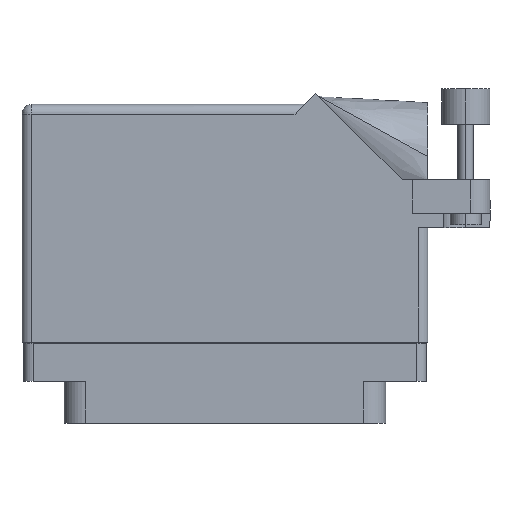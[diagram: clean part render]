
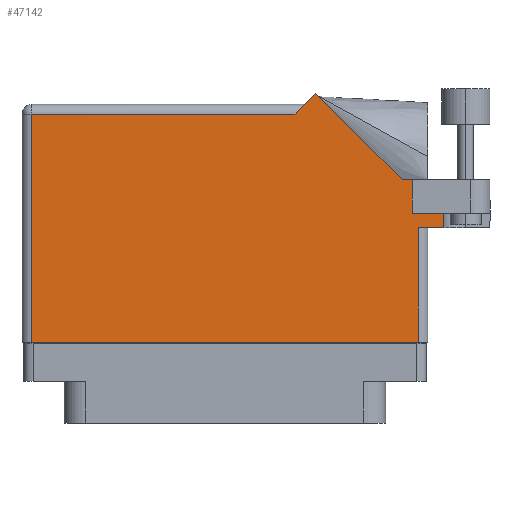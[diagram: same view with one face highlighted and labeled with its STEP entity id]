
A CAD part, front view. The second image highlights one B-rep face of the part: STEP entity #47142.
In plain terms, the highlighted face is planar.
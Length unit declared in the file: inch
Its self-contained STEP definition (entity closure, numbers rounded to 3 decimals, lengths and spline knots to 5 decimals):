
#153 = CARTESIAN_POINT ( 'NONE',  ( 1.206, 0.731, 0.455 ) ) ;
#438 = VERTEX_POINT ( 'NONE', #41555 ) ;
#1408 = LINE ( 'NONE', #45483, #38787 ) ;
#1766 = ORIENTED_EDGE ( 'NONE', *, *, #2080, .F. ) ;
#2080 = EDGE_CURVE ( 'NONE', #27989, #13766, #20685, .T. ) ;
#2596 = LINE ( 'NONE', #15896, #49463 ) ;
#3850 = VECTOR ( 'NONE', #30652, 39.37008 ) ;
#4051 = CARTESIAN_POINT ( 'NONE',  ( -1.244, 1.368, 0.455 ) ) ;
#4260 = EDGE_CURVE ( 'NONE', #438, #21775, #40558, .T. ) ;
#4798 = DIRECTION ( 'NONE',  ( 0., 0., -1. ) ) ;
#4998 = DIRECTION ( 'NONE',  ( -1., 0., 0. ) ) ;
#6506 = VECTOR ( 'NONE', #30229, 39.37008 ) ;
#7377 = LINE ( 'NONE', #37562, #49171 ) ;
#8509 = VERTEX_POINT ( 'NONE', #31426 ) ;
#9942 = EDGE_CURVE ( 'NONE', #13766, #21775, #1408, .T. ) ;
#10241 = VERTEX_POINT ( 'NONE', #4051 ) ;
#10254 = LINE ( 'NONE', #26733, #33143 ) ;
#10369 = CARTESIAN_POINT ( 'NONE',  ( -1.306, 1.368, 0.455 ) ) ;
#10616 = CARTESIAN_POINT ( 'NONE',  ( 1.14042, 0.944, 0.455 ) ) ;
#10882 = EDGE_CURVE ( 'NONE', #38971, #8509, #43104, .T. ) ;
#10927 = CARTESIAN_POINT ( 'NONE',  ( 0.451, 1.368, 0.455 ) ) ;
#11291 = EDGE_CURVE ( 'NONE', #8509, #37565, #29175, .T. ) ;
#12112 = ORIENTED_EDGE ( 'NONE', *, *, #28509, .T. ) ;
#13766 = VERTEX_POINT ( 'NONE', #40806 ) ;
#15241 = EDGE_CURVE ( 'NONE', #31106, #37190, #10254, .T. ) ;
#15896 = CARTESIAN_POINT ( 'NONE',  ( 1.244, 0.637, 0.455 ) ) ;
#17010 = DIRECTION ( 'NONE',  ( -1., 0., 0. ) ) ;
#17446 = CARTESIAN_POINT ( 'NONE',  ( 1.4075, 0.637, 0.455 ) ) ;
#17551 = DIRECTION ( 'NONE',  ( 1., 0., 0. ) ) ;
#18924 = VERTEX_POINT ( 'NONE', #46451 ) ;
#19337 = EDGE_CURVE ( 'NONE', #18924, #38971, #7377, .T. ) ;
#20122 = ORIENTED_EDGE ( 'NONE', *, *, #4260, .T. ) ;
#20175 = CARTESIAN_POINT ( 'NONE',  ( 1.244, -0.1, 0.455 ) ) ;
#20685 = LINE ( 'NONE', #153, #29537 ) ;
#21068 = ORIENTED_EDGE ( 'NONE', *, *, #10882, .T. ) ;
#21775 = VERTEX_POINT ( 'NONE', #17446 ) ;
#22113 = CARTESIAN_POINT ( 'NONE',  ( 1.306, 0.637, 0.455 ) ) ;
#22409 = LINE ( 'NONE', #50147, #35077 ) ;
#22490 = ORIENTED_EDGE ( 'NONE', *, *, #49039, .T. ) ;
#25108 = FACE_OUTER_BOUND ( 'NONE', #49254, .T. ) ;
#26733 = CARTESIAN_POINT ( 'NONE',  ( -1.306, -0.1, 0.455 ) ) ;
#27034 = ORIENTED_EDGE ( 'NONE', *, *, #48606, .T. ) ;
#27145 = ORIENTED_EDGE ( 'NONE', *, *, #9942, .F. ) ;
#27573 = DIRECTION ( 'NONE',  ( -0.707, -0.707, 0. ) ) ;
#27989 = VERTEX_POINT ( 'NONE', #44814 ) ;
#28123 = LINE ( 'NONE', #10369, #6506 ) ;
#28509 = EDGE_CURVE ( 'NONE', #37190, #438, #2596, .T. ) ;
#28562 = EDGE_CURVE ( 'NONE', #27989, #18924, #51931, .T. ) ;
#29175 = LINE ( 'NONE', #50712, #31028 ) ;
#29537 = VECTOR ( 'NONE', #36063, 39.37008 ) ;
#30229 = DIRECTION ( 'NONE',  ( -1., 0., 0. ) ) ;
#30652 = DIRECTION ( 'NONE',  ( -0.707, 0.707, 0. ) ) ;
#31028 = VECTOR ( 'NONE', #27573, 39.37008 ) ;
#31106 = VERTEX_POINT ( 'NONE', #38903 ) ;
#31426 = CARTESIAN_POINT ( 'NONE',  ( 0.58371, 1.50071, 0.455 ) ) ;
#31856 = DIRECTION ( 'NONE',  ( 0., 1., 0. ) ) ;
#32403 = CARTESIAN_POINT ( 'NONE',  ( 1.206, 0.731, 0.455 ) ) ;
#33143 = VECTOR ( 'NONE', #36094, 39.37008 ) ;
#35077 = VECTOR ( 'NONE', #38162, 39.37008 ) ;
#35736 = ORIENTED_EDGE ( 'NONE', *, *, #19337, .T. ) ;
#36063 = DIRECTION ( 'NONE',  ( 1., 0., 0. ) ) ;
#36094 = DIRECTION ( 'NONE',  ( 1., 0., 0. ) ) ;
#36137 = VECTOR ( 'NONE', #44573, 39.37008 ) ;
#37190 = VERTEX_POINT ( 'NONE', #20175 ) ;
#37562 = CARTESIAN_POINT ( 'NONE',  ( 1.706, 0.944, 0.455 ) ) ;
#37565 = VERTEX_POINT ( 'NONE', #10927 ) ;
#38162 = DIRECTION ( 'NONE',  ( 0., -1., 0. ) ) ;
#38787 = VECTOR ( 'NONE', #41062, 39.37008 ) ;
#38903 = CARTESIAN_POINT ( 'NONE',  ( -1.244, -0.1, 0.455 ) ) ;
#38971 = VERTEX_POINT ( 'NONE', #49530 ) ;
#40558 = LINE ( 'NONE', #22113, #49431 ) ;
#40806 = CARTESIAN_POINT ( 'NONE',  ( 1.4075, 0.731, 0.455 ) ) ;
#41062 = DIRECTION ( 'NONE',  ( 0., -1., 0. ) ) ;
#41555 = CARTESIAN_POINT ( 'NONE',  ( 1.244, 0.637, 0.455 ) ) ;
#43104 = LINE ( 'NONE', #10616, #3850 ) ;
#44075 = ORIENTED_EDGE ( 'NONE', *, *, #28562, .T. ) ;
#44573 = DIRECTION ( 'NONE',  ( 0., 1., 0. ) ) ;
#44802 = CARTESIAN_POINT ( 'NONE',  ( -1.306, 1.43, 0.455 ) ) ;
#44814 = CARTESIAN_POINT ( 'NONE',  ( 1.206, 0.731, 0.455 ) ) ;
#45112 = AXIS2_PLACEMENT_3D ( 'NONE', #44802, #4798, #17010 ) ;
#45483 = CARTESIAN_POINT ( 'NONE',  ( 1.4075, 1.06177, 0.455 ) ) ;
#46451 = CARTESIAN_POINT ( 'NONE',  ( 1.206, 0.944, 0.455 ) ) ;
#46603 = ORIENTED_EDGE ( 'NONE', *, *, #15241, .T. ) ;
#47142 = ADVANCED_FACE ( 'NONE', ( #25108 ), #49019, .F. ) ;
#48606 = EDGE_CURVE ( 'NONE', #10241, #31106, #22409, .T. ) ;
#49019 = PLANE ( 'NONE',  #45112 ) ;
#49039 = EDGE_CURVE ( 'NONE', #37565, #10241, #28123, .T. ) ;
#49171 = VECTOR ( 'NONE', #4998, 39.37008 ) ;
#49254 = EDGE_LOOP ( 'NONE', ( #46603, #12112, #20122, #27145, #1766, #44075, #35736, #21068, #49972, #22490, #27034 ) ) ;
#49431 = VECTOR ( 'NONE', #17551, 39.37008 ) ;
#49463 = VECTOR ( 'NONE', #31856, 39.37008 ) ;
#49530 = CARTESIAN_POINT ( 'NONE',  ( 1.14042, 0.944, 0.455 ) ) ;
#49972 = ORIENTED_EDGE ( 'NONE', *, *, #11291, .T. ) ;
#50147 = CARTESIAN_POINT ( 'NONE',  ( -1.244, -0.1, 0.455 ) ) ;
#50712 = CARTESIAN_POINT ( 'NONE',  ( 0.513, 1.43, 0.455 ) ) ;
#51931 = LINE ( 'NONE', #32403, #36137 ) ;
